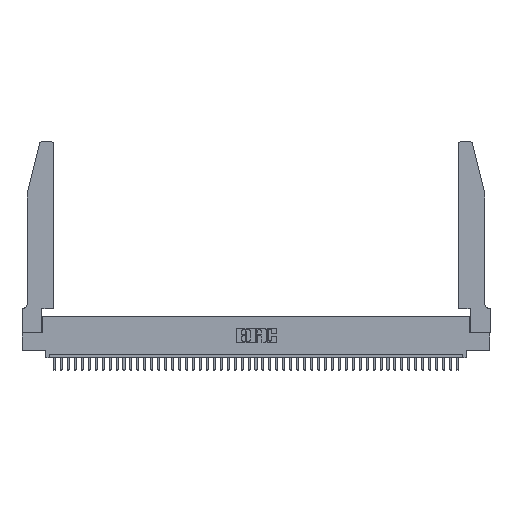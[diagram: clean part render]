
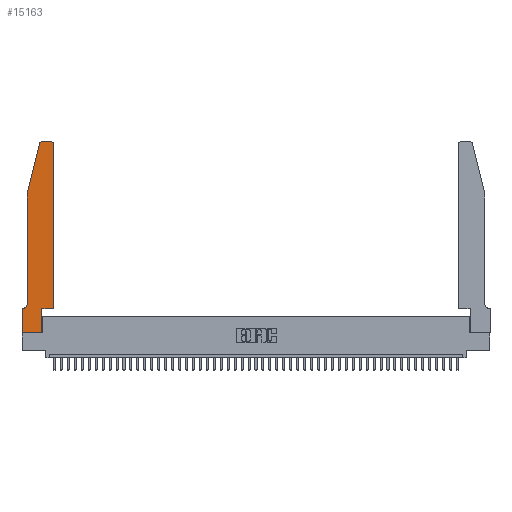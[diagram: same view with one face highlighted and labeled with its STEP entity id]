
A CAD part, top view. The second image highlights one B-rep face of the part: STEP entity #15163.
In plain terms, the highlighted planar face has unit normal (0, 0, 1).
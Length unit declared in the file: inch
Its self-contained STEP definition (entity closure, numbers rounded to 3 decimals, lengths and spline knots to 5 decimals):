
#320 = DIRECTION ( 'NONE',  ( 0., 1., 0. ) ) ;
#660 = VECTOR ( 'NONE', #19851, 39.37008 ) ;
#1229 = CARTESIAN_POINT ( 'NONE',  ( 0.0755, 0.35, 0.37 ) ) ;
#1857 = CIRCLE ( 'NONE', #4221, 0.07 ) ;
#3516 = LINE ( 'NONE', #3711, #38815 ) ;
#3711 = CARTESIAN_POINT ( 'NONE',  ( 0.4505, 0.35, 0.37 ) ) ;
#3777 = CARTESIAN_POINT ( 'NONE',  ( 0.0055, 0.42, 0.37 ) ) ;
#4221 = AXIS2_PLACEMENT_3D ( 'NONE', #3777, #39877, #21823 ) ;
#4624 = LINE ( 'NONE', #19237, #660 ) ;
#5877 = ORIENTED_EDGE ( 'NONE', *, *, #41439, .T. ) ;
#6264 = CARTESIAN_POINT ( 'NONE',  ( 0.4205, 2.72, 0.37 ) ) ;
#6716 = CARTESIAN_POINT ( 'NONE',  ( 0.0055, 0.35, 0.37 ) ) ;
#7233 = ORIENTED_EDGE ( 'NONE', *, *, #18802, .T. ) ;
#7658 = VERTEX_POINT ( 'NONE', #40917 ) ;
#7687 = DIRECTION ( 'NONE',  ( 1., 0., 0. ) ) ;
#8419 = CARTESIAN_POINT ( 'NONE',  ( 0.4205, 2.75, 0.37 ) ) ;
#12040 = EDGE_LOOP ( 'NONE', ( #21324, #7233, #38707, #42278, #14058, #19848, #5877, #32037, #30700, #29721, #42591, #24394 ) ) ;
#12149 = VERTEX_POINT ( 'NONE', #40532 ) ;
#12242 = EDGE_CURVE ( 'NONE', #7658, #12149, #28660, .T. ) ;
#12858 = EDGE_CURVE ( 'NONE', #12149, #28651, #4624, .T. ) ;
#13967 = DIRECTION ( 'NONE',  ( 0., 0., 1. ) ) ;
#14030 = CARTESIAN_POINT ( 'NONE',  ( 0.0755, 2., 0.37 ) ) ;
#14058 = ORIENTED_EDGE ( 'NONE', *, *, #28845, .T. ) ;
#14326 = AXIS2_PLACEMENT_3D ( 'NONE', #6264, #32396, #21288 ) ;
#14404 = LINE ( 'NONE', #23083, #34339 ) ;
#14505 = CARTESIAN_POINT ( 'NONE',  ( 0.4505, 2.72, 0.37 ) ) ;
#15052 = CARTESIAN_POINT ( 'NONE',  ( 0.4505, 0.35, 0.37 ) ) ;
#15072 = DIRECTION ( 'NONE',  ( 0., 0., 1. ) ) ;
#15163 = ADVANCED_FACE ( 'NONE', ( #31709 ), #28617, .T. ) ;
#15182 = EDGE_CURVE ( 'NONE', #28868, #34725, #46422, .T. ) ;
#17340 = VERTEX_POINT ( 'NONE', #30310 ) ;
#17608 = DIRECTION ( 'NONE',  ( 1., 0., 0. ) ) ;
#18332 = CARTESIAN_POINT ( 'NONE',  ( 0.0755, 2., 0.37 ) ) ;
#18802 = EDGE_CURVE ( 'NONE', #37054, #21460, #23356, .T. ) ;
#18823 = CARTESIAN_POINT ( 'NONE',  ( 0.4505, 0.35, 0.37 ) ) ;
#18982 = DIRECTION ( 'NONE',  ( 1., 0., 0. ) ) ;
#19237 = CARTESIAN_POINT ( 'NONE',  ( 0.2865, 0.35, 0.37 ) ) ;
#19259 = DIRECTION ( 'NONE',  ( -1., 0., 0. ) ) ;
#19620 = EDGE_CURVE ( 'NONE', #23242, #28868, #34176, .T. ) ;
#19848 = ORIENTED_EDGE ( 'NONE', *, *, #42414, .T. ) ;
#19851 = DIRECTION ( 'NONE',  ( 0., 1., 0. ) ) ;
#21288 = DIRECTION ( 'NONE',  ( 1., 0., 0. ) ) ;
#21324 = ORIENTED_EDGE ( 'NONE', *, *, #44520, .T. ) ;
#21460 = VERTEX_POINT ( 'NONE', #25369 ) ;
#21769 = VECTOR ( 'NONE', #24687, 39.37008 ) ;
#21823 = DIRECTION ( 'NONE',  ( -1., 0., 0. ) ) ;
#22899 = LINE ( 'NONE', #14030, #21769 ) ;
#22940 = EDGE_CURVE ( 'NONE', #21460, #38675, #22899, .T. ) ;
#23083 = CARTESIAN_POINT ( 'NONE',  ( 0.2605, 2.75, 0.37 ) ) ;
#23242 = VERTEX_POINT ( 'NONE', #15052 ) ;
#23356 = CIRCLE ( 'NONE', #45152, 0.03 ) ;
#23793 = LINE ( 'NONE', #25209, #41963 ) ;
#24394 = ORIENTED_EDGE ( 'NONE', *, *, #15182, .T. ) ;
#24687 = DIRECTION ( 'NONE',  ( -0.239, -0.971, 0. ) ) ;
#25209 = CARTESIAN_POINT ( 'NONE',  ( 0., 0., 0.37 ) ) ;
#25369 = CARTESIAN_POINT ( 'NONE',  ( 0.25487, 2.72718, 0.37 ) ) ;
#25398 = VECTOR ( 'NONE', #19259, 39.37008 ) ;
#26746 = CARTESIAN_POINT ( 'NONE',  ( 0., 0., 0.37 ) ) ;
#28607 = VECTOR ( 'NONE', #18982, 39.37008 ) ;
#28617 = PLANE ( 'NONE',  #39560 ) ;
#28651 = VERTEX_POINT ( 'NONE', #40654 ) ;
#28660 = LINE ( 'NONE', #26746, #28607 ) ;
#28689 = CARTESIAN_POINT ( 'NONE',  ( 0.0755, 2., 0.37 ) ) ;
#28845 = EDGE_CURVE ( 'NONE', #17340, #35550, #1857, .T. ) ;
#28868 = VERTEX_POINT ( 'NONE', #14505 ) ;
#29721 = ORIENTED_EDGE ( 'NONE', *, *, #34595, .T. ) ;
#29854 = CARTESIAN_POINT ( 'NONE',  ( 0.284, 2.72, 0.37 ) ) ;
#30310 = CARTESIAN_POINT ( 'NONE',  ( 0.0755, 0.42, 0.37 ) ) ;
#30700 = ORIENTED_EDGE ( 'NONE', *, *, #12858, .T. ) ;
#31709 = FACE_OUTER_BOUND ( 'NONE', #12040, .T. ) ;
#32037 = ORIENTED_EDGE ( 'NONE', *, *, #12242, .T. ) ;
#32396 = DIRECTION ( 'NONE',  ( 0., 0., 1. ) ) ;
#33003 = DIRECTION ( 'NONE',  ( 1., 0., 0. ) ) ;
#33156 = VERTEX_POINT ( 'NONE', #46613 ) ;
#34176 = LINE ( 'NONE', #18823, #43222 ) ;
#34339 = VECTOR ( 'NONE', #41324, 39.37008 ) ;
#34595 = EDGE_CURVE ( 'NONE', #28651, #23242, #3516, .T. ) ;
#34725 = VERTEX_POINT ( 'NONE', #8419 ) ;
#35423 = CARTESIAN_POINT ( 'NONE',  ( 0., 0.35, 0.37 ) ) ;
#35550 = VERTEX_POINT ( 'NONE', #6716 ) ;
#36287 = DIRECTION ( 'NONE',  ( 0., -1., 0. ) ) ;
#36416 = LINE ( 'NONE', #28689, #42618 ) ;
#37054 = VERTEX_POINT ( 'NONE', #45562 ) ;
#38675 = VERTEX_POINT ( 'NONE', #18332 ) ;
#38707 = ORIENTED_EDGE ( 'NONE', *, *, #22940, .T. ) ;
#38815 = VECTOR ( 'NONE', #7687, 39.37008 ) ;
#39560 = AXIS2_PLACEMENT_3D ( 'NONE', #35423, #13967, #17608 ) ;
#39877 = DIRECTION ( 'NONE',  ( 0., 0., -1. ) ) ;
#40374 = EDGE_CURVE ( 'NONE', #38675, #17340, #36416, .T. ) ;
#40532 = CARTESIAN_POINT ( 'NONE',  ( 0.2865, 0., 0.37 ) ) ;
#40654 = CARTESIAN_POINT ( 'NONE',  ( 0.2865, 0.35, 0.37 ) ) ;
#40917 = CARTESIAN_POINT ( 'NONE',  ( 0., 0., 0.37 ) ) ;
#41324 = DIRECTION ( 'NONE',  ( -1., 0., 0. ) ) ;
#41439 = EDGE_CURVE ( 'NONE', #33156, #7658, #23793, .T. ) ;
#41963 = VECTOR ( 'NONE', #43449, 39.37008 ) ;
#42278 = ORIENTED_EDGE ( 'NONE', *, *, #40374, .T. ) ;
#42414 = EDGE_CURVE ( 'NONE', #35550, #33156, #42998, .T. ) ;
#42591 = ORIENTED_EDGE ( 'NONE', *, *, #19620, .T. ) ;
#42618 = VECTOR ( 'NONE', #36287, 39.37008 ) ;
#42998 = LINE ( 'NONE', #1229, #25398 ) ;
#43222 = VECTOR ( 'NONE', #320, 39.37008 ) ;
#43449 = DIRECTION ( 'NONE',  ( 0., -1., 0. ) ) ;
#44520 = EDGE_CURVE ( 'NONE', #34725, #37054, #14404, .T. ) ;
#45152 = AXIS2_PLACEMENT_3D ( 'NONE', #29854, #15072, #33003 ) ;
#45562 = CARTESIAN_POINT ( 'NONE',  ( 0.284, 2.75, 0.37 ) ) ;
#46422 = CIRCLE ( 'NONE', #14326, 0.03 ) ;
#46613 = CARTESIAN_POINT ( 'NONE',  ( 0., 0.35, 0.37 ) ) ;
